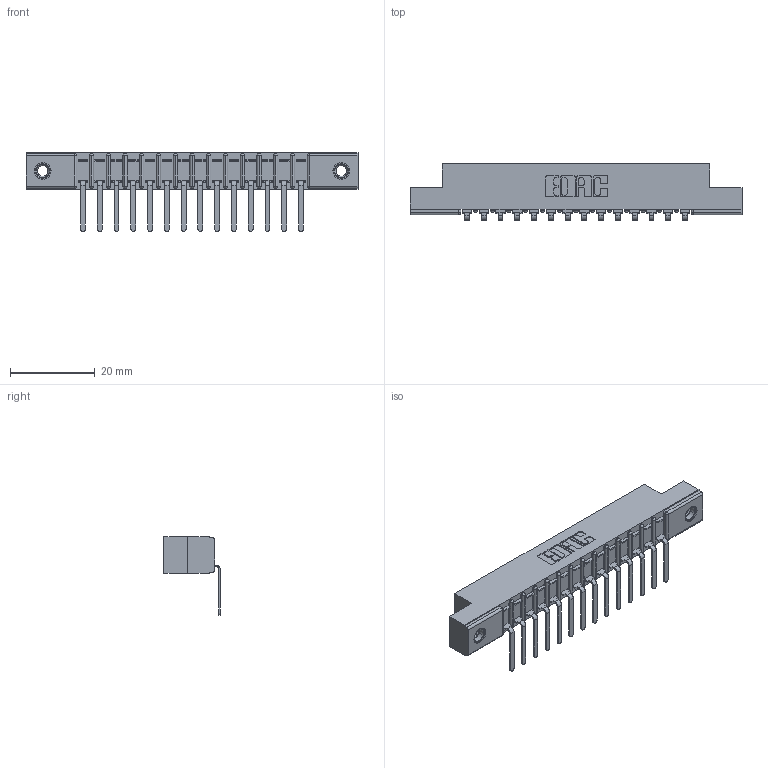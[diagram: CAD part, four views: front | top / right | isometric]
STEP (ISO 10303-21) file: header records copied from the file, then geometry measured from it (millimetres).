
FILE_DESCRIPTION (( 'STEP AP203' ), '1' );
FILE_NAME ('307-014-457-107.STEP', '2020-09-25T16:15:09', ( '' ), ( '' ), 'SwSTEP 2.0', 'SolidWorks 2020', '' );
FILE_SCHEMA (( 'CONFIG_CONTROL_DESIGN' ));
Length unit declared in the file: inch
Products named in the file (4): 307 Part_.156 Dia Mounting Holes; 307-014-457-107; 307-290-002_557; 345-250-001_345-250-005-103
Assembly tree (17 placements, depth 2):
  307-014-457-107
    307 Part_.156 Dia Mounting Holes
    307-290-002_557  x14
    345-250-001_345-250-005-103  x2
Bounding box: 78.49 x 13.32 x 18.67 mm (x, y, z)
Volume: 5201.6 mm3; surface area: 9282.4 mm2
Topology: 17 solids, 17 shells, 1285 faces, 3875 edges, 2534 vertices
Faces by surface type: plane 760, cylinder 479, sphere 30, cone 12, torus 4
Entity records: 17493 total; most frequent: CARTESIAN_POINT 2927, ORIENTED_EDGE 2910, DIRECTION 2867, EDGE_CURVE 1455, VECTOR 1099, LINE 1099, VERTEX_POINT 944, AXIS2_PLACEMENT_3D 884
